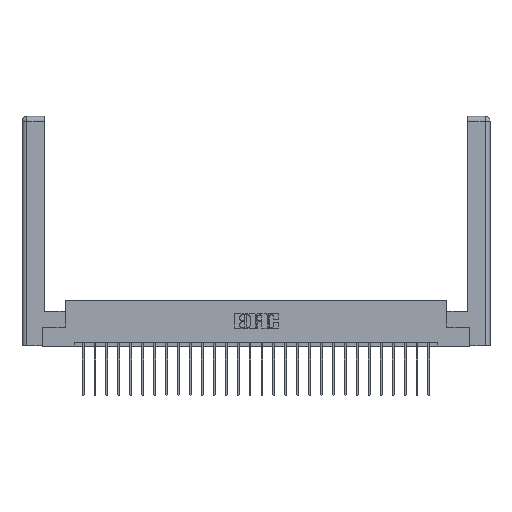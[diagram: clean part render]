
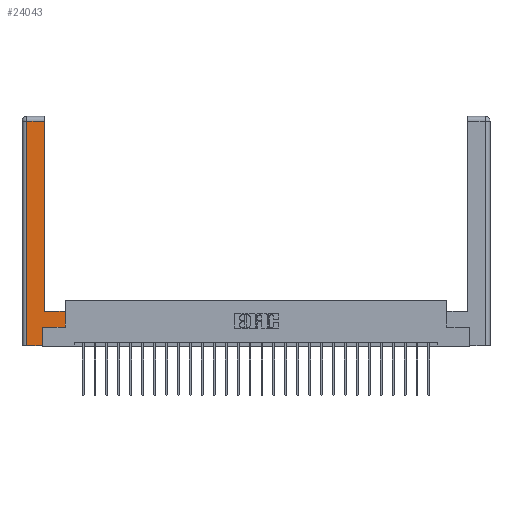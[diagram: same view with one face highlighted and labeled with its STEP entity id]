
A CAD part, top view. The second image highlights one B-rep face of the part: STEP entity #24043.
In plain terms, the highlighted planar face has unit normal (0, 0, 1).
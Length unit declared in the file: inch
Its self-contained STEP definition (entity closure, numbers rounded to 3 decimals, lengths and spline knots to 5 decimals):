
#748 = VECTOR ( 'NONE', #24459, 39.37008 ) ;
#926 = VECTOR ( 'NONE', #15391, 39.37008 ) ;
#946 = ORIENTED_EDGE ( 'NONE', *, *, #10566, .T. ) ;
#1389 = EDGE_CURVE ( 'NONE', #20670, #24774, #24165, .T. ) ;
#1400 = DIRECTION ( 'NONE',  ( -1., 0., 0. ) ) ;
#1409 = LINE ( 'NONE', #24197, #748 ) ;
#1587 = DIRECTION ( 'NONE',  ( -1., 0., 0. ) ) ;
#2436 = ORIENTED_EDGE ( 'NONE', *, *, #2944, .T. ) ;
#2588 = AXIS2_PLACEMENT_3D ( 'NONE', #18022, #26452, #1587 ) ;
#2771 = CARTESIAN_POINT ( 'NONE',  ( 0.295, 3., 0. ) ) ;
#2846 = LINE ( 'NONE', #11181, #17753 ) ;
#2944 = EDGE_CURVE ( 'NONE', #22542, #22923, #2846, .T. ) ;
#3475 = CARTESIAN_POINT ( 'NONE',  ( 0.0615, 0., 0. ) ) ;
#3768 = CARTESIAN_POINT ( 'NONE',  ( 0.0615, 0., 0. ) ) ;
#4348 = EDGE_CURVE ( 'NONE', #22923, #17050, #1409, .T. ) ;
#4568 = ORIENTED_EDGE ( 'NONE', *, *, #27025, .T. ) ;
#5862 = CARTESIAN_POINT ( 'NONE',  ( 0.565, 0.245, 0. ) ) ;
#5874 = ORIENTED_EDGE ( 'NONE', *, *, #4348, .T. ) ;
#7172 = ORIENTED_EDGE ( 'NONE', *, *, #22676, .T. ) ;
#8825 = FACE_OUTER_BOUND ( 'NONE', #13181, .T. ) ;
#9016 = VECTOR ( 'NONE', #20322, 39.37008 ) ;
#10523 = DIRECTION ( 'NONE',  ( 1., 0., 0. ) ) ;
#10566 = EDGE_CURVE ( 'NONE', #14425, #26593, #15569, .T. ) ;
#10633 = LINE ( 'NONE', #24871, #15262 ) ;
#10786 = ORIENTED_EDGE ( 'NONE', *, *, #15105, .T. ) ;
#11150 = ORIENTED_EDGE ( 'NONE', *, *, #1389, .T. ) ;
#11181 = CARTESIAN_POINT ( 'NONE',  ( 0.565, 0.245, 0. ) ) ;
#12141 = CARTESIAN_POINT ( 'NONE',  ( 0.295, 2.94, 0. ) ) ;
#12524 = VECTOR ( 'NONE', #10523, 39.37008 ) ;
#13181 = EDGE_LOOP ( 'NONE', ( #946, #4568, #24623, #11150, #7172, #2436, #5874, #10786 ) ) ;
#13342 = CARTESIAN_POINT ( 'NONE',  ( 0.265, 0.245, 0. ) ) ;
#13617 = LINE ( 'NONE', #23299, #24275 ) ;
#13853 = CARTESIAN_POINT ( 'NONE',  ( 0.295, 0.45, 0. ) ) ;
#14295 = PLANE ( 'NONE',  #2588 ) ;
#14425 = VERTEX_POINT ( 'NONE', #13853 ) ;
#14819 = EDGE_CURVE ( 'NONE', #19428, #20670, #24960, .T. ) ;
#15105 = EDGE_CURVE ( 'NONE', #17050, #14425, #13617, .T. ) ;
#15262 = VECTOR ( 'NONE', #1400, 39.37008 ) ;
#15391 = DIRECTION ( 'NONE',  ( 0., 1., 0. ) ) ;
#15569 = LINE ( 'NONE', #2771, #17919 ) ;
#16976 = DIRECTION ( 'NONE',  ( -1., 0., 0. ) ) ;
#17050 = VERTEX_POINT ( 'NONE', #21800 ) ;
#17753 = VECTOR ( 'NONE', #26298, 39.37008 ) ;
#17919 = VECTOR ( 'NONE', #19646, 39.37008 ) ;
#18022 = CARTESIAN_POINT ( 'NONE',  ( 0., 0., 0. ) ) ;
#19428 = VERTEX_POINT ( 'NONE', #26888 ) ;
#19646 = DIRECTION ( 'NONE',  ( 0., 1., 0. ) ) ;
#20322 = DIRECTION ( 'NONE',  ( 0., -1., 0. ) ) ;
#20670 = VERTEX_POINT ( 'NONE', #3768 ) ;
#20929 = CARTESIAN_POINT ( 'NONE',  ( 0.265, 0., 0. ) ) ;
#21800 = CARTESIAN_POINT ( 'NONE',  ( 0.565, 0.45, 0. ) ) ;
#22542 = VERTEX_POINT ( 'NONE', #23865 ) ;
#22676 = EDGE_CURVE ( 'NONE', #24774, #22542, #24176, .T. ) ;
#22913 = CARTESIAN_POINT ( 'NONE',  ( 0.265, 0., 0. ) ) ;
#22923 = VERTEX_POINT ( 'NONE', #5862 ) ;
#23299 = CARTESIAN_POINT ( 'NONE',  ( 0.295, 0.45, 0. ) ) ;
#23865 = CARTESIAN_POINT ( 'NONE',  ( 0.265, 0.245, 0. ) ) ;
#24043 = ADVANCED_FACE ( 'NONE', ( #8825 ), #14295, .F. ) ;
#24165 = LINE ( 'NONE', #20929, #12524 ) ;
#24176 = LINE ( 'NONE', #13342, #926 ) ;
#24197 = CARTESIAN_POINT ( 'NONE',  ( 0.565, 0.45, 0. ) ) ;
#24275 = VECTOR ( 'NONE', #16976, 39.37008 ) ;
#24459 = DIRECTION ( 'NONE',  ( 0., 1., 0. ) ) ;
#24623 = ORIENTED_EDGE ( 'NONE', *, *, #14819, .T. ) ;
#24774 = VERTEX_POINT ( 'NONE', #22913 ) ;
#24871 = CARTESIAN_POINT ( 'NONE',  ( 0.0615, 2.94, 0. ) ) ;
#24960 = LINE ( 'NONE', #3475, #9016 ) ;
#26298 = DIRECTION ( 'NONE',  ( 1., 0., 0. ) ) ;
#26452 = DIRECTION ( 'NONE',  ( 0., 0., -1. ) ) ;
#26593 = VERTEX_POINT ( 'NONE', #12141 ) ;
#26888 = CARTESIAN_POINT ( 'NONE',  ( 0.0615, 2.94, 0. ) ) ;
#27025 = EDGE_CURVE ( 'NONE', #26593, #19428, #10633, .T. ) ;
